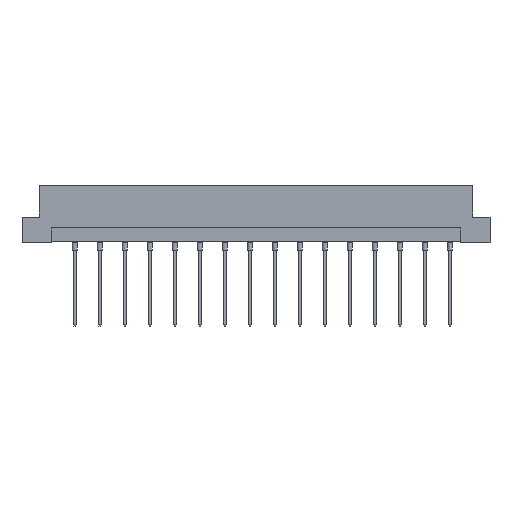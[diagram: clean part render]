
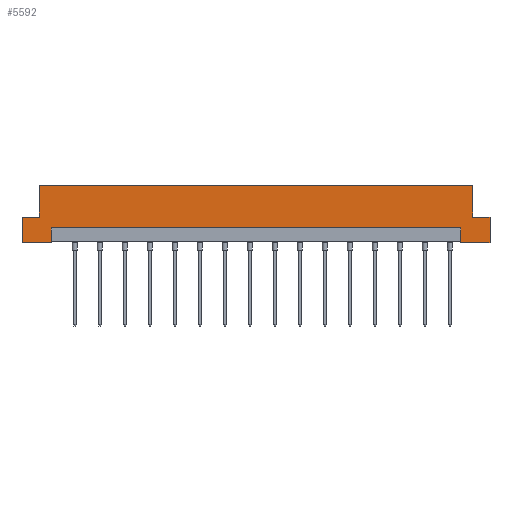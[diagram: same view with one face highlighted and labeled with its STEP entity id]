
A CAD part, front view. The second image highlights one B-rep face of the part: STEP entity #5592.
In plain terms, the highlighted planar face has unit normal (0, -1, 0).
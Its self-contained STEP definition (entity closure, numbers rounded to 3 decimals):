
#46 = CARTESIAN_POINT ( 'NONE',  ( -44., -4.3, 11.6 ) ) ;
#88 = LINE ( 'NONE', #6344, #9575 ) ;
#126 = CARTESIAN_POINT ( 'NONE',  ( 44., -4.3, 5.2 ) ) ;
#452 = VERTEX_POINT ( 'NONE', #7284 ) ;
#523 = EDGE_CURVE ( 'NONE', #3368, #7522, #10956, .T. ) ;
#569 = ORIENTED_EDGE ( 'NONE', *, *, #9802, .T. ) ;
#667 = DIRECTION ( 'NONE',  ( 0., 1., 0. ) ) ;
#704 = CARTESIAN_POINT ( 'NONE',  ( 41.6, -4.3, 0.2 ) ) ;
#834 = CARTESIAN_POINT ( 'NONE',  ( -47.5, -4.3, 5.2 ) ) ;
#890 = VECTOR ( 'NONE', #5713, 1000. ) ;
#1029 = LINE ( 'NONE', #4590, #3013 ) ;
#1243 = DIRECTION ( 'NONE',  ( 0., 0., -1. ) ) ;
#1283 = VECTOR ( 'NONE', #5490, 1000. ) ;
#1434 = CARTESIAN_POINT ( 'NONE',  ( -41.6, -4.3, 3. ) ) ;
#1446 = VECTOR ( 'NONE', #4104, 1000. ) ;
#1522 = CARTESIAN_POINT ( 'NONE',  ( 47.5, -4.3, 0. ) ) ;
#1640 = VECTOR ( 'NONE', #1805, 1000. ) ;
#1657 = EDGE_CURVE ( 'NONE', #3219, #3958, #2459, .T. ) ;
#1701 = CARTESIAN_POINT ( 'NONE',  ( -44., -4.3, 5.2 ) ) ;
#1805 = DIRECTION ( 'NONE',  ( 1., 0., 0. ) ) ;
#1853 = LINE ( 'NONE', #9154, #10674 ) ;
#2102 = CARTESIAN_POINT ( 'NONE',  ( 47.5, -4.3, 0. ) ) ;
#2179 = ORIENTED_EDGE ( 'NONE', *, *, #8068, .F. ) ;
#2207 = VERTEX_POINT ( 'NONE', #46 ) ;
#2381 = EDGE_CURVE ( 'NONE', #452, #3958, #6595, .T. ) ;
#2459 = LINE ( 'NONE', #704, #8543 ) ;
#2516 = LINE ( 'NONE', #6958, #1640 ) ;
#2639 = ORIENTED_EDGE ( 'NONE', *, *, #8841, .T. ) ;
#2871 = VERTEX_POINT ( 'NONE', #11248 ) ;
#2874 = VERTEX_POINT ( 'NONE', #1701 ) ;
#3013 = VECTOR ( 'NONE', #3705, 1000. ) ;
#3068 = VERTEX_POINT ( 'NONE', #6440 ) ;
#3219 = VERTEX_POINT ( 'NONE', #10341 ) ;
#3368 = VERTEX_POINT ( 'NONE', #5196 ) ;
#3418 = CARTESIAN_POINT ( 'NONE',  ( 47.5, -4.3, 11.6 ) ) ;
#3705 = DIRECTION ( 'NONE',  ( 1., 0., 0. ) ) ;
#3958 = VERTEX_POINT ( 'NONE', #5351 ) ;
#3991 = LINE ( 'NONE', #9132, #10444 ) ;
#4082 = EDGE_CURVE ( 'NONE', #2207, #3068, #1029, .T. ) ;
#4104 = DIRECTION ( 'NONE',  ( 1., 0., 0. ) ) ;
#4112 = VERTEX_POINT ( 'NONE', #6638 ) ;
#4338 = VECTOR ( 'NONE', #8095, 1000. ) ;
#4590 = CARTESIAN_POINT ( 'NONE',  ( 47.5, -4.3, 11.6 ) ) ;
#4616 = EDGE_CURVE ( 'NONE', #452, #2871, #3991, .T. ) ;
#4676 = ORIENTED_EDGE ( 'NONE', *, *, #4082, .F. ) ;
#5196 = CARTESIAN_POINT ( 'NONE',  ( 47.5, -4.3, 5.2 ) ) ;
#5351 = CARTESIAN_POINT ( 'NONE',  ( 41.6, -4.3, 3. ) ) ;
#5490 = DIRECTION ( 'NONE',  ( 0., 0., 1. ) ) ;
#5592 = ADVANCED_FACE ( 'NONE', ( #7755 ), #8676, .F. ) ;
#5624 = LINE ( 'NONE', #126, #6983 ) ;
#5713 = DIRECTION ( 'NONE',  ( 1., 0., 0. ) ) ;
#5964 = CARTESIAN_POINT ( 'NONE',  ( -47.5, -4.3, 0. ) ) ;
#5966 = EDGE_CURVE ( 'NONE', #4112, #3068, #5624, .T. ) ;
#6344 = CARTESIAN_POINT ( 'NONE',  ( -47.5, -4.3, 11.6 ) ) ;
#6440 = CARTESIAN_POINT ( 'NONE',  ( 44., -4.3, 11.6 ) ) ;
#6595 = LINE ( 'NONE', #1434, #890 ) ;
#6638 = CARTESIAN_POINT ( 'NONE',  ( 44., -4.3, 5.2 ) ) ;
#6958 = CARTESIAN_POINT ( 'NONE',  ( 47.5, -4.3, 0. ) ) ;
#6983 = VECTOR ( 'NONE', #8259, 1000. ) ;
#7021 = DIRECTION ( 'NONE',  ( 0., 0., 1. ) ) ;
#7284 = CARTESIAN_POINT ( 'NONE',  ( -41.6, -4.3, 3. ) ) ;
#7522 = VERTEX_POINT ( 'NONE', #1522 ) ;
#7548 = AXIS2_PLACEMENT_3D ( 'NONE', #3418, #667, #11310 ) ;
#7638 = VECTOR ( 'NONE', #10142, 1000. ) ;
#7682 = ORIENTED_EDGE ( 'NONE', *, *, #10538, .F. ) ;
#7755 = FACE_OUTER_BOUND ( 'NONE', #8733, .T. ) ;
#8068 = EDGE_CURVE ( 'NONE', #8887, #2874, #1853, .T. ) ;
#8081 = ORIENTED_EDGE ( 'NONE', *, *, #4616, .F. ) ;
#8095 = DIRECTION ( 'NONE',  ( 1., 0., 0. ) ) ;
#8126 = ORIENTED_EDGE ( 'NONE', *, *, #5966, .T. ) ;
#8259 = DIRECTION ( 'NONE',  ( 0., 0., 1. ) ) ;
#8264 = ORIENTED_EDGE ( 'NONE', *, *, #11340, .F. ) ;
#8543 = VECTOR ( 'NONE', #7021, 1000. ) ;
#8676 = PLANE ( 'NONE',  #7548 ) ;
#8717 = LINE ( 'NONE', #9644, #1446 ) ;
#8733 = EDGE_LOOP ( 'NONE', ( #10322, #11321, #2639, #11335, #7682, #8126, #4676, #8264, #2179, #569, #9055, #8081 ) ) ;
#8841 = EDGE_CURVE ( 'NONE', #3219, #7522, #10162, .T. ) ;
#8887 = VERTEX_POINT ( 'NONE', #834 ) ;
#9055 = ORIENTED_EDGE ( 'NONE', *, *, #11140, .T. ) ;
#9132 = CARTESIAN_POINT ( 'NONE',  ( -41.6, -4.3, 0.2 ) ) ;
#9154 = CARTESIAN_POINT ( 'NONE',  ( -47.5, -4.3, 5.2 ) ) ;
#9575 = VECTOR ( 'NONE', #10774, 1000. ) ;
#9644 = CARTESIAN_POINT ( 'NONE',  ( 47.5, -4.3, 5.2 ) ) ;
#9802 = EDGE_CURVE ( 'NONE', #8887, #10985, #88, .T. ) ;
#10079 = CARTESIAN_POINT ( 'NONE',  ( 47.5, -4.3, 11.6 ) ) ;
#10142 = DIRECTION ( 'NONE',  ( 0., 0., -1. ) ) ;
#10162 = LINE ( 'NONE', #2102, #4338 ) ;
#10322 = ORIENTED_EDGE ( 'NONE', *, *, #2381, .T. ) ;
#10341 = CARTESIAN_POINT ( 'NONE',  ( 41.6, -4.3, 0. ) ) ;
#10444 = VECTOR ( 'NONE', #1243, 1000. ) ;
#10538 = EDGE_CURVE ( 'NONE', #4112, #3368, #8717, .T. ) ;
#10674 = VECTOR ( 'NONE', #10733, 1000. ) ;
#10733 = DIRECTION ( 'NONE',  ( 1., 0., 0. ) ) ;
#10774 = DIRECTION ( 'NONE',  ( 0., 0., -1. ) ) ;
#10922 = CARTESIAN_POINT ( 'NONE',  ( -44., -4.3, 5.2 ) ) ;
#10956 = LINE ( 'NONE', #10079, #7638 ) ;
#10985 = VERTEX_POINT ( 'NONE', #5964 ) ;
#11034 = LINE ( 'NONE', #10922, #1283 ) ;
#11140 = EDGE_CURVE ( 'NONE', #10985, #2871, #2516, .T. ) ;
#11248 = CARTESIAN_POINT ( 'NONE',  ( -41.6, -4.3, 0. ) ) ;
#11310 = DIRECTION ( 'NONE',  ( -1., 0., 0. ) ) ;
#11321 = ORIENTED_EDGE ( 'NONE', *, *, #1657, .F. ) ;
#11335 = ORIENTED_EDGE ( 'NONE', *, *, #523, .F. ) ;
#11340 = EDGE_CURVE ( 'NONE', #2874, #2207, #11034, .T. ) ;
